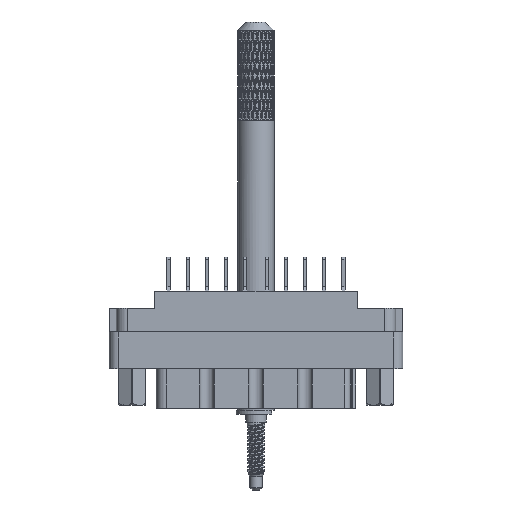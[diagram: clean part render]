
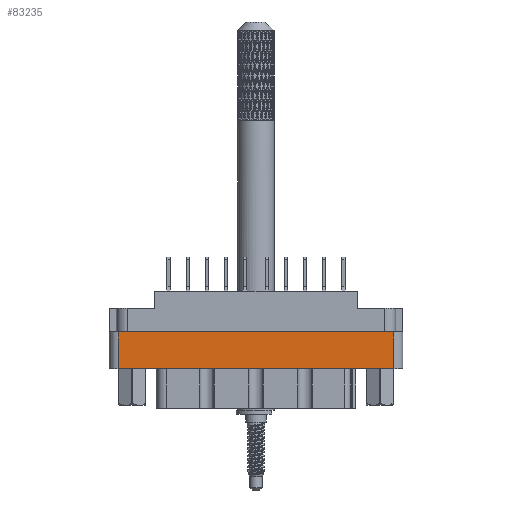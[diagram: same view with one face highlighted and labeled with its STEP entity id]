
A CAD part, front view. The second image highlights one B-rep face of the part: STEP entity #83235.
In plain terms, the highlighted planar face has unit normal (0, -1, 0).
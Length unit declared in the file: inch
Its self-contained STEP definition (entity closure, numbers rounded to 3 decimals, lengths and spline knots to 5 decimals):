
#2449 = ORIENTED_EDGE ( 'NONE', *, *, #61219, .F. ) ;
#4174 = CARTESIAN_POINT ( 'NONE',  ( -0.938, -0.438, -0.798 ) ) ;
#4936 = DIRECTION ( 'NONE',  ( 0., 0., -1. ) ) ;
#8518 = LINE ( 'NONE', #4174, #98705 ) ;
#9314 = EDGE_LOOP ( 'NONE', ( #2449, #81264, #20642, #84100 ) ) ;
#9625 = LINE ( 'NONE', #28915, #34221 ) ;
#12845 = DIRECTION ( 'NONE',  ( 0., 0., -1. ) ) ;
#13232 = LINE ( 'NONE', #106573, #62410 ) ;
#20642 = ORIENTED_EDGE ( 'NONE', *, *, #63662, .F. ) ;
#21285 = CARTESIAN_POINT ( 'NONE',  ( -1., -0.438, -0.798 ) ) ;
#27341 = AXIS2_PLACEMENT_3D ( 'NONE', #21285, #92248, #12845 ) ;
#28915 = CARTESIAN_POINT ( 'NONE',  ( 0., -0.438, -0.277 ) ) ;
#33219 = VERTEX_POINT ( 'NONE', #39979 ) ;
#33825 = CARTESIAN_POINT ( 'NONE',  ( -0.938, -0.438, -0.277 ) ) ;
#34221 = VECTOR ( 'NONE', #89980, 39.37008 ) ;
#36569 = VERTEX_POINT ( 'NONE', #33825 ) ;
#39816 = VECTOR ( 'NONE', #111695, 39.37008 ) ;
#39979 = CARTESIAN_POINT ( 'NONE',  ( 0.938, -0.438, -0.277 ) ) ;
#40921 = CARTESIAN_POINT ( 'NONE',  ( 0.938, -0.438, -0.529 ) ) ;
#41772 = CARTESIAN_POINT ( 'NONE',  ( 0.938, -0.438, -0.798 ) ) ;
#43074 = CARTESIAN_POINT ( 'NONE',  ( -0.938, -0.438, -0.529 ) ) ;
#51939 = EDGE_CURVE ( 'NONE', #36569, #81372, #8518, .T. ) ;
#56108 = LINE ( 'NONE', #41772, #39816 ) ;
#60511 = VERTEX_POINT ( 'NONE', #40921 ) ;
#61219 = EDGE_CURVE ( 'NONE', #36569, #33219, #9625, .T. ) ;
#62410 = VECTOR ( 'NONE', #97406, 39.37008 ) ;
#63662 = EDGE_CURVE ( 'NONE', #60511, #81372, #13232, .T. ) ;
#68977 = FACE_OUTER_BOUND ( 'NONE', #9314, .T. ) ;
#71386 = EDGE_CURVE ( 'NONE', #60511, #33219, #56108, .T. ) ;
#81264 = ORIENTED_EDGE ( 'NONE', *, *, #51939, .T. ) ;
#81372 = VERTEX_POINT ( 'NONE', #43074 ) ;
#83235 = ADVANCED_FACE ( 'NONE', ( #68977 ), #101086, .T. ) ;
#84100 = ORIENTED_EDGE ( 'NONE', *, *, #71386, .T. ) ;
#89980 = DIRECTION ( 'NONE',  ( 1., 0., 0. ) ) ;
#92248 = DIRECTION ( 'NONE',  ( 0., -1., 0. ) ) ;
#97406 = DIRECTION ( 'NONE',  ( -1., 0., 0. ) ) ;
#98705 = VECTOR ( 'NONE', #4936, 39.37008 ) ;
#101086 = PLANE ( 'NONE',  #27341 ) ;
#106573 = CARTESIAN_POINT ( 'NONE',  ( 0., -0.438, -0.529 ) ) ;
#111695 = DIRECTION ( 'NONE',  ( 0., 0., 1. ) ) ;
